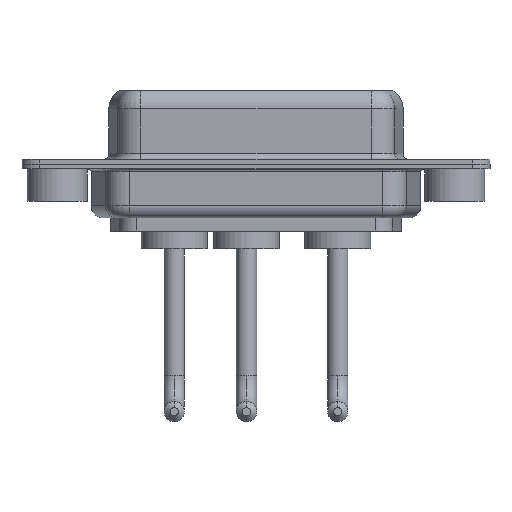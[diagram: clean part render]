
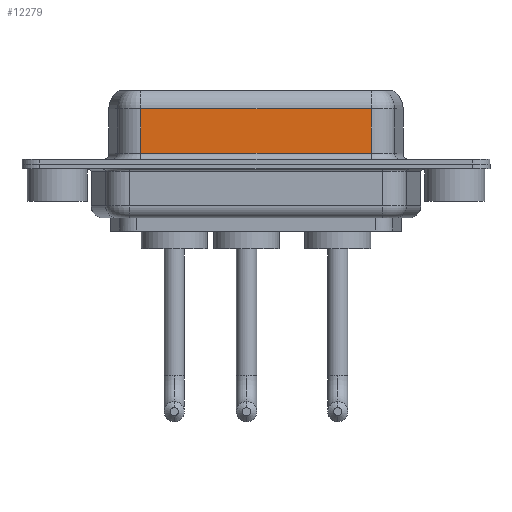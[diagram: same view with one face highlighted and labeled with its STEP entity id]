
A CAD part, front view. The second image highlights one B-rep face of the part: STEP entity #12279.
In plain terms, the highlighted planar face has unit normal (0, -1, 0).
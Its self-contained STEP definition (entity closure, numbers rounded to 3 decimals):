
#84 = EDGE_CURVE ( 'NONE', #4466, #9371, #2846, .T. ) ;
#205 = DIRECTION ( 'NONE',  ( 0., 0., -1. ) ) ;
#489 = DIRECTION ( 'NONE',  ( 0., 1., 0. ) ) ;
#530 = VECTOR ( 'NONE', #1942, 1000. ) ;
#651 = VECTOR ( 'NONE', #9754, 1000. ) ;
#912 = CARTESIAN_POINT ( 'NONE',  ( 26.287, -3.95, 6.4 ) ) ;
#1172 = CARTESIAN_POINT ( 'NONE',  ( 26.287, -3.95, 0.9 ) ) ;
#1180 = DIRECTION ( 'NONE',  ( 0., 0., -1. ) ) ;
#1377 = CARTESIAN_POINT ( 'NONE',  ( 26.287, -3.95, 4.65 ) ) ;
#1460 = FACE_OUTER_BOUND ( 'NONE', #1714, .T. ) ;
#1714 = EDGE_LOOP ( 'NONE', ( #4846, #11629, #3863, #12623 ) ) ;
#1942 = DIRECTION ( 'NONE',  ( 1., 0., 0. ) ) ;
#2499 = DIRECTION ( 'NONE',  ( 0., 0., 1. ) ) ;
#2842 = VECTOR ( 'NONE', #1180, 1000. ) ;
#2846 = LINE ( 'NONE', #13585, #530 ) ;
#3395 = CARTESIAN_POINT ( 'NONE',  ( 26.287, -3.95, 4.65 ) ) ;
#3863 = ORIENTED_EDGE ( 'NONE', *, *, #6202, .T. ) ;
#4466 = VERTEX_POINT ( 'NONE', #12208 ) ;
#4505 = CARTESIAN_POINT ( 'NONE',  ( 26.287, -3.95, 6.4 ) ) ;
#4846 = ORIENTED_EDGE ( 'NONE', *, *, #6127, .F. ) ;
#6127 = EDGE_CURVE ( 'NONE', #9346, #9371, #6171, .T. ) ;
#6171 = LINE ( 'NONE', #912, #2842 ) ;
#6174 = AXIS2_PLACEMENT_3D ( 'NONE', #4505, #489, #2499 ) ;
#6202 = EDGE_CURVE ( 'NONE', #9636, #4466, #13084, .T. ) ;
#7394 = CARTESIAN_POINT ( 'NONE',  ( 7.013, -3.95, 4.65 ) ) ;
#7574 = LINE ( 'NONE', #3395, #651 ) ;
#8180 = VECTOR ( 'NONE', #205, 1000. ) ;
#8744 = CARTESIAN_POINT ( 'NONE',  ( 7.013, -3.95, 6.4 ) ) ;
#9346 = VERTEX_POINT ( 'NONE', #1377 ) ;
#9371 = VERTEX_POINT ( 'NONE', #1172 ) ;
#9636 = VERTEX_POINT ( 'NONE', #7394 ) ;
#9754 = DIRECTION ( 'NONE',  ( -1., 0., 0. ) ) ;
#10025 = PLANE ( 'NONE',  #6174 ) ;
#11051 = EDGE_CURVE ( 'NONE', #9346, #9636, #7574, .T. ) ;
#11629 = ORIENTED_EDGE ( 'NONE', *, *, #11051, .T. ) ;
#12208 = CARTESIAN_POINT ( 'NONE',  ( 7.013, -3.95, 0.9 ) ) ;
#12279 = ADVANCED_FACE ( 'NONE', ( #1460 ), #10025, .F. ) ;
#12623 = ORIENTED_EDGE ( 'NONE', *, *, #84, .T. ) ;
#13084 = LINE ( 'NONE', #8744, #8180 ) ;
#13585 = CARTESIAN_POINT ( 'NONE',  ( 26.287, -3.95, 0.9 ) ) ;
